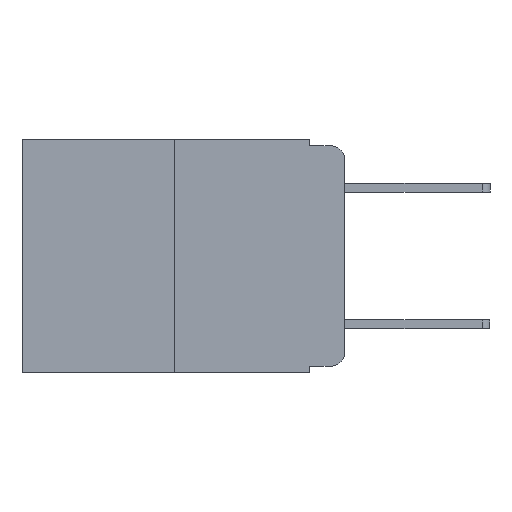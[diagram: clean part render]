
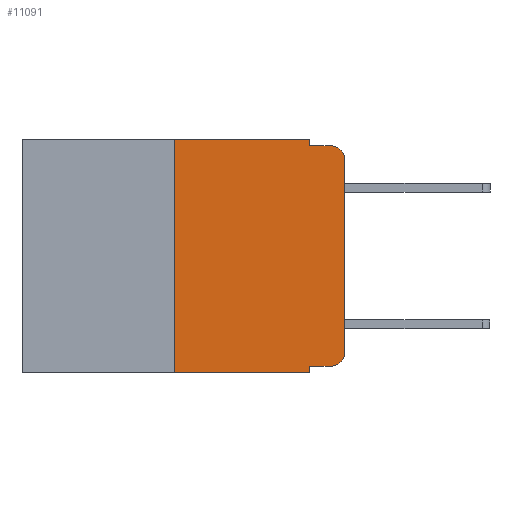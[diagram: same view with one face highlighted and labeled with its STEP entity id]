
A CAD part, left-side view. The second image highlights one B-rep face of the part: STEP entity #11091.
In plain terms, the highlighted planar face has unit normal (-1, 0, 0).
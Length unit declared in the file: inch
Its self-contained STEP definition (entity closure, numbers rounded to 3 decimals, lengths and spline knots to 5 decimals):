
#423 = EDGE_CURVE ( 'NONE', #5813, #15588, #7418, .T. ) ;
#931 = VERTEX_POINT ( 'NONE', #8096 ) ;
#1494 = LINE ( 'NONE', #5910, #9451 ) ;
#1688 = ORIENTED_EDGE ( 'NONE', *, *, #2020, .T. ) ;
#1797 = VERTEX_POINT ( 'NONE', #11458 ) ;
#1855 = VECTOR ( 'NONE', #10518, 39.37008 ) ;
#1969 = DIRECTION ( 'NONE',  ( 0., 0., -1. ) ) ;
#2020 = EDGE_CURVE ( 'NONE', #5509, #5813, #11985, .T. ) ;
#2031 = CARTESIAN_POINT ( 'NONE',  ( 0., 0.051, -0.343 ) ) ;
#2062 = LINE ( 'NONE', #6867, #13829 ) ;
#2137 = VERTEX_POINT ( 'NONE', #11804 ) ;
#2337 = CARTESIAN_POINT ( 'NONE',  ( 0., 0.25, -0.343 ) ) ;
#2497 = LINE ( 'NONE', #12249, #18088 ) ;
#3033 = CARTESIAN_POINT ( 'NONE',  ( 0., 0.051, -0.333 ) ) ;
#3050 = DIRECTION ( 'NONE',  ( 0., -1., 0. ) ) ;
#3201 = ORIENTED_EDGE ( 'NONE', *, *, #13867, .F. ) ;
#3739 = CIRCLE ( 'NONE', #6677, 0.02 ) ;
#3747 = ORIENTED_EDGE ( 'NONE', *, *, #16891, .F. ) ;
#4730 = EDGE_CURVE ( 'NONE', #2137, #931, #12113, .T. ) ;
#4783 = VECTOR ( 'NONE', #15251, 39.37008 ) ;
#4897 = VERTEX_POINT ( 'NONE', #2031 ) ;
#5209 = CARTESIAN_POINT ( 'NONE',  ( 0., 0.02, -0.03 ) ) ;
#5332 = EDGE_CURVE ( 'NONE', #8375, #5509, #12787, .T. ) ;
#5407 = AXIS2_PLACEMENT_3D ( 'NONE', #11500, #12603, #12534 ) ;
#5509 = VERTEX_POINT ( 'NONE', #6761 ) ;
#5813 = VERTEX_POINT ( 'NONE', #11819 ) ;
#5910 = CARTESIAN_POINT ( 'NONE',  ( 0., 0.051, 0. ) ) ;
#6020 = DIRECTION ( 'NONE',  ( 0., 0., 1. ) ) ;
#6136 = EDGE_LOOP ( 'NONE', ( #13930, #10932, #3201, #3747, #16650, #12567, #9607, #13943, #16460, #1688 ) ) ;
#6459 = VECTOR ( 'NONE', #18242, 39.37008 ) ;
#6677 = AXIS2_PLACEMENT_3D ( 'NONE', #5209, #15650, #6783 ) ;
#6761 = CARTESIAN_POINT ( 'NONE',  ( 0., 0.02, -0.333 ) ) ;
#6783 = DIRECTION ( 'NONE',  ( 0., 0., -1. ) ) ;
#6867 = CARTESIAN_POINT ( 'NONE',  ( 0., 0.051, 0. ) ) ;
#7418 = LINE ( 'NONE', #18304, #6459 ) ;
#7461 = DIRECTION ( 'NONE',  ( 0., 0., -1. ) ) ;
#7504 = CARTESIAN_POINT ( 'NONE',  ( 0., 0.25, 0. ) ) ;
#7538 = EDGE_CURVE ( 'NONE', #13737, #4897, #2497, .T. ) ;
#7983 = DIRECTION ( 'NONE',  ( 0., 0., -1. ) ) ;
#8064 = EDGE_CURVE ( 'NONE', #13737, #2137, #9415, .T. ) ;
#8096 = CARTESIAN_POINT ( 'NONE',  ( 0., 0.051, 0. ) ) ;
#8164 = CARTESIAN_POINT ( 'NONE',  ( 0., 0.02, -0.01 ) ) ;
#8219 = VECTOR ( 'NONE', #15336, 39.37008 ) ;
#8375 = VERTEX_POINT ( 'NONE', #15681 ) ;
#9083 = CARTESIAN_POINT ( 'NONE',  ( 0., 0.051, -0.01 ) ) ;
#9415 = LINE ( 'NONE', #7504, #12845 ) ;
#9451 = VECTOR ( 'NONE', #7461, 39.37008 ) ;
#9481 = EDGE_CURVE ( 'NONE', #15588, #19543, #3739, .T. ) ;
#9607 = ORIENTED_EDGE ( 'NONE', *, *, #7538, .T. ) ;
#10208 = LINE ( 'NONE', #9083, #1855 ) ;
#10518 = DIRECTION ( 'NONE',  ( 0., -1., 0. ) ) ;
#10932 = ORIENTED_EDGE ( 'NONE', *, *, #9481, .T. ) ;
#11091 = ADVANCED_FACE ( 'NONE', ( #17288 ), #13833, .F. ) ;
#11448 = AXIS2_PLACEMENT_3D ( 'NONE', #19610, #16748, #7983 ) ;
#11458 = CARTESIAN_POINT ( 'NONE',  ( 0., 0.051, -0.01 ) ) ;
#11500 = CARTESIAN_POINT ( 'NONE',  ( 0., 0.02, -0.313 ) ) ;
#11753 = CARTESIAN_POINT ( 'NONE',  ( 0., 0., -0.03 ) ) ;
#11804 = CARTESIAN_POINT ( 'NONE',  ( 0., 0.25, 0. ) ) ;
#11819 = CARTESIAN_POINT ( 'NONE',  ( 0., 0., -0.313 ) ) ;
#11985 = CIRCLE ( 'NONE', #5407, 0.02 ) ;
#12113 = LINE ( 'NONE', #12322, #8219 ) ;
#12249 = CARTESIAN_POINT ( 'NONE',  ( 0., 0.473, -0.343 ) ) ;
#12322 = CARTESIAN_POINT ( 'NONE',  ( 0., 0.473, 0. ) ) ;
#12387 = EDGE_CURVE ( 'NONE', #8375, #4897, #2062, .T. ) ;
#12534 = DIRECTION ( 'NONE',  ( 0., 0., -1. ) ) ;
#12567 = ORIENTED_EDGE ( 'NONE', *, *, #8064, .F. ) ;
#12603 = DIRECTION ( 'NONE',  ( -1., 0., 0. ) ) ;
#12787 = LINE ( 'NONE', #3033, #4783 ) ;
#12845 = VECTOR ( 'NONE', #6020, 39.37008 ) ;
#13737 = VERTEX_POINT ( 'NONE', #2337 ) ;
#13829 = VECTOR ( 'NONE', #1969, 39.37008 ) ;
#13833 = PLANE ( 'NONE',  #11448 ) ;
#13867 = EDGE_CURVE ( 'NONE', #1797, #19543, #10208, .T. ) ;
#13930 = ORIENTED_EDGE ( 'NONE', *, *, #423, .T. ) ;
#13943 = ORIENTED_EDGE ( 'NONE', *, *, #12387, .F. ) ;
#15251 = DIRECTION ( 'NONE',  ( 0., -1., 0. ) ) ;
#15336 = DIRECTION ( 'NONE',  ( 0., -1., 0. ) ) ;
#15588 = VERTEX_POINT ( 'NONE', #11753 ) ;
#15650 = DIRECTION ( 'NONE',  ( -1., 0., 0. ) ) ;
#15681 = CARTESIAN_POINT ( 'NONE',  ( 0., 0.051, -0.333 ) ) ;
#16460 = ORIENTED_EDGE ( 'NONE', *, *, #5332, .T. ) ;
#16650 = ORIENTED_EDGE ( 'NONE', *, *, #4730, .F. ) ;
#16748 = DIRECTION ( 'NONE',  ( 1., 0., 0. ) ) ;
#16891 = EDGE_CURVE ( 'NONE', #931, #1797, #1494, .T. ) ;
#17288 = FACE_OUTER_BOUND ( 'NONE', #6136, .T. ) ;
#18088 = VECTOR ( 'NONE', #3050, 39.37008 ) ;
#18242 = DIRECTION ( 'NONE',  ( 0., 0., 1. ) ) ;
#18304 = CARTESIAN_POINT ( 'NONE',  ( 0., 0., 0. ) ) ;
#19543 = VERTEX_POINT ( 'NONE', #8164 ) ;
#19610 = CARTESIAN_POINT ( 'NONE',  ( 0., 0.473, 0. ) ) ;
